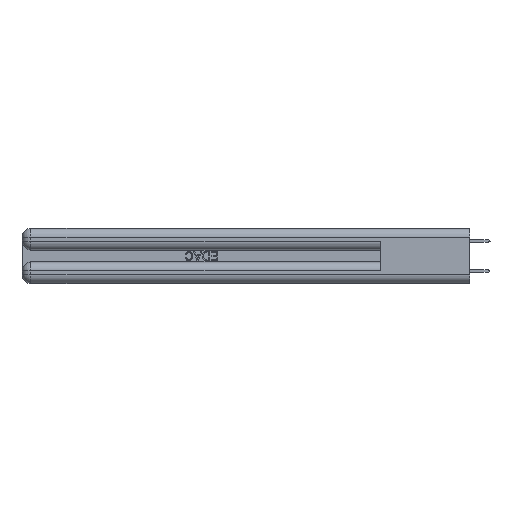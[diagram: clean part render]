
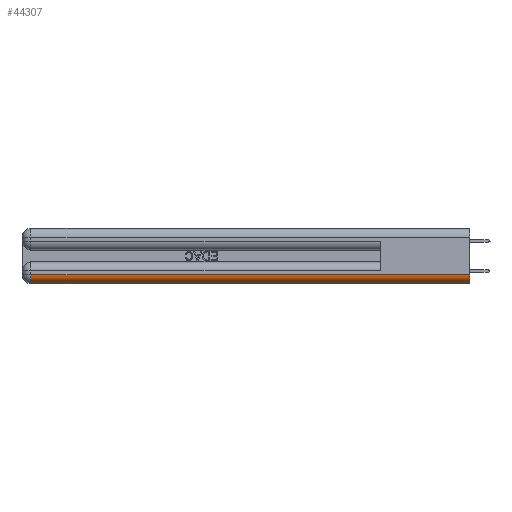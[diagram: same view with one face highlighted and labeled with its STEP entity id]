
A CAD part, left-side view. The second image highlights one B-rep face of the part: STEP entity #44307.
In plain terms, the highlighted cylindrical face has radius 1.524 mm (diameter 3.048 mm), a partial arc.
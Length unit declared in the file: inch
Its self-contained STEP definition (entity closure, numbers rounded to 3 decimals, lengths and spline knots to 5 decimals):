
#2008 = CARTESIAN_POINT ( 'NONE',  ( 0.06, 0., 0. ) ) ;
#2600 = CARTESIAN_POINT ( 'NONE',  ( 0.06, 2.94, 0.06 ) ) ;
#3865 = DIRECTION ( 'NONE',  ( 0., -1., 0. ) ) ;
#5739 = EDGE_CURVE ( 'NONE', #16476, #7096, #45956, .T. ) ;
#6350 = EDGE_CURVE ( 'NONE', #7096, #40264, #42870, .T. ) ;
#7096 = VERTEX_POINT ( 'NONE', #37554 ) ;
#7967 = ORIENTED_EDGE ( 'NONE', *, *, #26090, .F. ) ;
#9265 = CARTESIAN_POINT ( 'NONE',  ( 0.06, 0., 0.06 ) ) ;
#10178 = DIRECTION ( 'NONE',  ( 0., 1., 0. ) ) ;
#12788 = DIRECTION ( 'NONE',  ( 0., 1., 0. ) ) ;
#12895 = CARTESIAN_POINT ( 'NONE',  ( 0.06, 0., 0.06 ) ) ;
#14932 = VERTEX_POINT ( 'NONE', #2008 ) ;
#16476 = VERTEX_POINT ( 'NONE', #21858 ) ;
#16528 = DIRECTION ( 'NONE',  ( 0., 1., 0. ) ) ;
#16960 = CARTESIAN_POINT ( 'NONE',  ( 0., 0., 0.06 ) ) ;
#17562 = CARTESIAN_POINT ( 'NONE',  ( 0., 0., 0.06 ) ) ;
#21858 = CARTESIAN_POINT ( 'NONE',  ( 0.06, 2.94, 0. ) ) ;
#23656 = CIRCLE ( 'NONE', #38018, 0.06 ) ;
#24087 = EDGE_LOOP ( 'NONE', ( #34261, #30127, #33437, #7967 ) ) ;
#25603 = AXIS2_PLACEMENT_3D ( 'NONE', #2600, #16528, #44908 ) ;
#26090 = EDGE_CURVE ( 'NONE', #14932, #16476, #42526, .T. ) ;
#27305 = DIRECTION ( 'NONE',  ( 0., -1., 0. ) ) ;
#30127 = ORIENTED_EDGE ( 'NONE', *, *, #6350, .F. ) ;
#33437 = ORIENTED_EDGE ( 'NONE', *, *, #5739, .F. ) ;
#34261 = ORIENTED_EDGE ( 'NONE', *, *, #39442, .F. ) ;
#34726 = VECTOR ( 'NONE', #3865, 39.37008 ) ;
#35408 = CARTESIAN_POINT ( 'NONE',  ( 0.06, 3., 0. ) ) ;
#37554 = CARTESIAN_POINT ( 'NONE',  ( 0., 2.94, 0.06 ) ) ;
#38018 = AXIS2_PLACEMENT_3D ( 'NONE', #12895, #27305, #45502 ) ;
#39442 = EDGE_CURVE ( 'NONE', #40264, #14932, #23656, .T. ) ;
#40264 = VERTEX_POINT ( 'NONE', #16960 ) ;
#41427 = VECTOR ( 'NONE', #10178, 39.37008 ) ;
#41613 = DIRECTION ( 'NONE',  ( 0., 0., 1. ) ) ;
#42526 = LINE ( 'NONE', #35408, #41427 ) ;
#42870 = LINE ( 'NONE', #17562, #34726 ) ;
#43997 = FACE_OUTER_BOUND ( 'NONE', #24087, .T. ) ;
#44307 = ADVANCED_FACE ( 'NONE', ( #43997 ), #45382, .T. ) ;
#44347 = AXIS2_PLACEMENT_3D ( 'NONE', #9265, #12788, #41613 ) ;
#44908 = DIRECTION ( 'NONE',  ( 0., 0., 1. ) ) ;
#45382 = CYLINDRICAL_SURFACE ( 'NONE', #44347, 0.06 ) ;
#45502 = DIRECTION ( 'NONE',  ( 0., 0., 1. ) ) ;
#45956 = CIRCLE ( 'NONE', #25603, 0.06 ) ;
